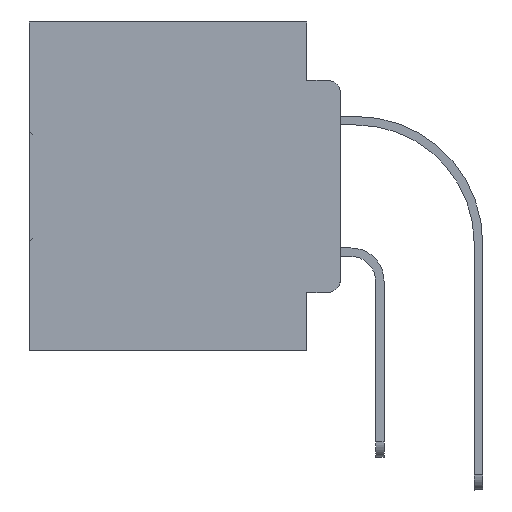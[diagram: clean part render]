
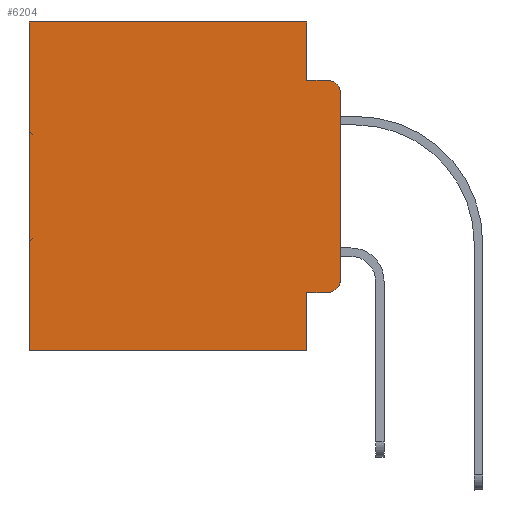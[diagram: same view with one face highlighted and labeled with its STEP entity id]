
A CAD part, left-side view. The second image highlights one B-rep face of the part: STEP entity #6204.
In plain terms, the highlighted planar face has unit normal (-1, 0, 0).
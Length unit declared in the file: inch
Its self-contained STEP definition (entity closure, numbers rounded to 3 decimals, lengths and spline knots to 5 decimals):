
#46 = DIRECTION ( 'NONE',  ( -1., 0., 0. ) ) ;
#269 = ORIENTED_EDGE ( 'NONE', *, *, #5853, .F. ) ;
#628 = LINE ( 'NONE', #12050, #1884 ) ;
#1884 = VECTOR ( 'NONE', #3816, 39.37008 ) ;
#2483 = DIRECTION ( 'NONE',  ( 0., 0., -1. ) ) ;
#2578 = DIRECTION ( 'NONE',  ( 0., -1., 0. ) ) ;
#3119 = VECTOR ( 'NONE', #20065, 39.37008 ) ;
#3816 = DIRECTION ( 'NONE',  ( 0., 1., 0. ) ) ;
#4098 = FACE_OUTER_BOUND ( 'NONE', #17448, .T. ) ;
#4160 = ORIENTED_EDGE ( 'NONE', *, *, #29408, .T. ) ;
#5210 = CARTESIAN_POINT ( 'NONE',  ( 0.298, 0.473, 0. ) ) ;
#5853 = EDGE_CURVE ( 'NONE', #33479, #29115, #22698, .T. ) ;
#6204 = ADVANCED_FACE ( 'NONE', ( #4098 ), #12911, .F. ) ;
#6510 = VERTEX_POINT ( 'NONE', #27292 ) ;
#7159 = CARTESIAN_POINT ( 'NONE',  ( 0.298, 0.473, 0. ) ) ;
#7204 = LINE ( 'NONE', #18624, #28599 ) ;
#7762 = DIRECTION ( 'NONE',  ( 0., 0., -1. ) ) ;
#7917 = VECTOR ( 'NONE', #2578, 39.37008 ) ;
#8299 = CARTESIAN_POINT ( 'NONE',  ( 0.298, 0.051, 0. ) ) ;
#8626 = CARTESIAN_POINT ( 'NONE',  ( 0.298, 0.051, -0.0885 ) ) ;
#8935 = EDGE_CURVE ( 'NONE', #27111, #35118, #20854, .T. ) ;
#10324 = VECTOR ( 'NONE', #2483, 39.37008 ) ;
#10329 = AXIS2_PLACEMENT_3D ( 'NONE', #12020, #46, #11467 ) ;
#10364 = CARTESIAN_POINT ( 'NONE',  ( 0.298, 0.02, -0.1085 ) ) ;
#11467 = DIRECTION ( 'NONE',  ( 0., 0., -1. ) ) ;
#12020 = CARTESIAN_POINT ( 'NONE',  ( 0.298, 0.02, -0.3915 ) ) ;
#12050 = CARTESIAN_POINT ( 'NONE',  ( 0.298, 0., 0. ) ) ;
#12072 = EDGE_CURVE ( 'NONE', #31517, #33479, #7204, .T. ) ;
#12464 = CARTESIAN_POINT ( 'NONE',  ( 0.298, 0.051, -0.4115 ) ) ;
#12911 = PLANE ( 'NONE',  #30090 ) ;
#12978 = DIRECTION ( 'NONE',  ( 0., 0., -1. ) ) ;
#13274 = DIRECTION ( 'NONE',  ( 0., 1., 0. ) ) ;
#13703 = AXIS2_PLACEMENT_3D ( 'NONE', #10364, #15255, #25365 ) ;
#14180 = DIRECTION ( 'NONE',  ( 0., 0., -1. ) ) ;
#14360 = CARTESIAN_POINT ( 'NONE',  ( 0.298, 0., 0. ) ) ;
#14600 = ORIENTED_EDGE ( 'NONE', *, *, #17231, .T. ) ;
#15031 = ORIENTED_EDGE ( 'NONE', *, *, #8935, .T. ) ;
#15255 = DIRECTION ( 'NONE',  ( -1., 0., 0. ) ) ;
#15530 = DIRECTION ( 'NONE',  ( 1., 0., 0. ) ) ;
#15792 = CARTESIAN_POINT ( 'NONE',  ( 0.298, 0., -0.1085 ) ) ;
#15825 = CARTESIAN_POINT ( 'NONE',  ( 0.298, 0.051, -0.0885 ) ) ;
#15856 = CARTESIAN_POINT ( 'NONE',  ( 0.298, 0.02, -0.4115 ) ) ;
#16096 = CARTESIAN_POINT ( 'NONE',  ( 0.298, 0., 0. ) ) ;
#16212 = VECTOR ( 'NONE', #14180, 39.37008 ) ;
#16311 = EDGE_CURVE ( 'NONE', #35715, #32442, #19919, .T. ) ;
#17231 = EDGE_CURVE ( 'NONE', #35715, #17599, #28251, .T. ) ;
#17448 = EDGE_LOOP ( 'NONE', ( #32661, #35021, #269, #28677, #25859, #15031, #23079, #22717, #14600, #4160 ) ) ;
#17599 = VERTEX_POINT ( 'NONE', #15856 ) ;
#18013 = CARTESIAN_POINT ( 'NONE',  ( 0.298, 0.051, 0. ) ) ;
#18374 = EDGE_CURVE ( 'NONE', #32442, #35118, #26769, .T. ) ;
#18472 = CIRCLE ( 'NONE', #13703, 0.02 ) ;
#18624 = CARTESIAN_POINT ( 'NONE',  ( 0.298, 0.051, 0. ) ) ;
#18998 = CARTESIAN_POINT ( 'NONE',  ( 0.298, 0.051, -0.5 ) ) ;
#19919 = LINE ( 'NONE', #8299, #10324 ) ;
#20065 = DIRECTION ( 'NONE',  ( 0., -1., 0. ) ) ;
#20854 = LINE ( 'NONE', #7159, #24010 ) ;
#21533 = CARTESIAN_POINT ( 'NONE',  ( 0.298, 0., -0.5 ) ) ;
#22698 = LINE ( 'NONE', #8626, #3119 ) ;
#22717 = ORIENTED_EDGE ( 'NONE', *, *, #16311, .F. ) ;
#23079 = ORIENTED_EDGE ( 'NONE', *, *, #18374, .F. ) ;
#24010 = VECTOR ( 'NONE', #12978, 39.37008 ) ;
#24100 = EDGE_CURVE ( 'NONE', #25995, #6510, #28229, .T. ) ;
#24652 = EDGE_CURVE ( 'NONE', #31517, #27111, #628, .T. ) ;
#25080 = CARTESIAN_POINT ( 'NONE',  ( 0.298, 0.051, -0.4115 ) ) ;
#25365 = DIRECTION ( 'NONE',  ( 0., 0., -1. ) ) ;
#25859 = ORIENTED_EDGE ( 'NONE', *, *, #24652, .T. ) ;
#25995 = VERTEX_POINT ( 'NONE', #15792 ) ;
#26515 = VECTOR ( 'NONE', #13274, 39.37008 ) ;
#26769 = LINE ( 'NONE', #21533, #26515 ) ;
#26960 = DIRECTION ( 'NONE',  ( 0., 0., -1. ) ) ;
#27111 = VERTEX_POINT ( 'NONE', #5210 ) ;
#27292 = CARTESIAN_POINT ( 'NONE',  ( 0.298, 0., -0.3915 ) ) ;
#27658 = CIRCLE ( 'NONE', #10329, 0.02 ) ;
#27905 = EDGE_CURVE ( 'NONE', #25995, #29115, #18472, .T. ) ;
#28229 = LINE ( 'NONE', #14360, #16212 ) ;
#28251 = LINE ( 'NONE', #25080, #7917 ) ;
#28599 = VECTOR ( 'NONE', #7762, 39.37008 ) ;
#28677 = ORIENTED_EDGE ( 'NONE', *, *, #12072, .F. ) ;
#29115 = VERTEX_POINT ( 'NONE', #30421 ) ;
#29408 = EDGE_CURVE ( 'NONE', #17599, #6510, #27658, .T. ) ;
#30090 = AXIS2_PLACEMENT_3D ( 'NONE', #16096, #15530, #26960 ) ;
#30421 = CARTESIAN_POINT ( 'NONE',  ( 0.298, 0.02, -0.0885 ) ) ;
#30754 = CARTESIAN_POINT ( 'NONE',  ( 0.298, 0.473, -0.5 ) ) ;
#31517 = VERTEX_POINT ( 'NONE', #18013 ) ;
#32442 = VERTEX_POINT ( 'NONE', #18998 ) ;
#32661 = ORIENTED_EDGE ( 'NONE', *, *, #24100, .F. ) ;
#33479 = VERTEX_POINT ( 'NONE', #15825 ) ;
#35021 = ORIENTED_EDGE ( 'NONE', *, *, #27905, .T. ) ;
#35118 = VERTEX_POINT ( 'NONE', #30754 ) ;
#35715 = VERTEX_POINT ( 'NONE', #12464 ) ;
